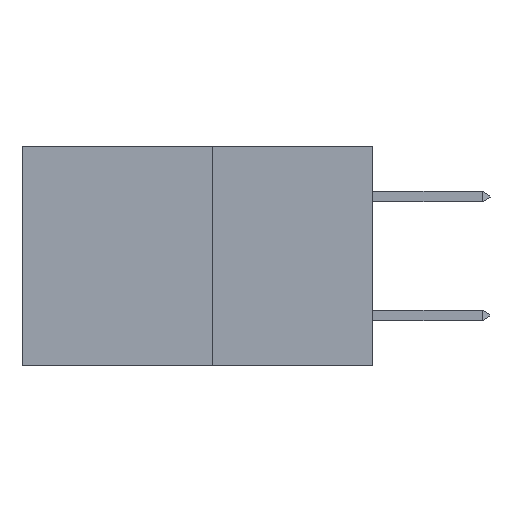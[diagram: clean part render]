
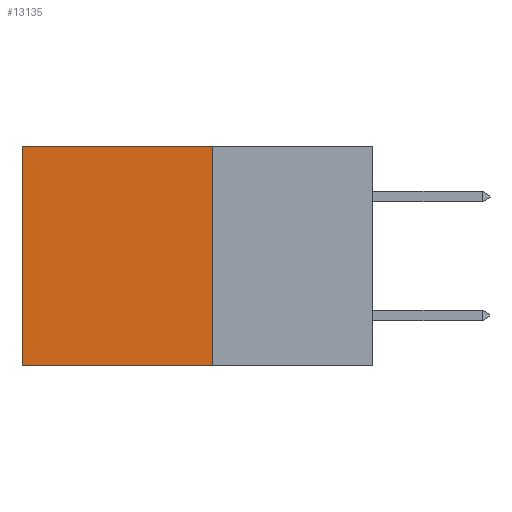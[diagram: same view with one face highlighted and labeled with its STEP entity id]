
A CAD part, left-side view. The second image highlights one B-rep face of the part: STEP entity #13135.
In plain terms, the highlighted planar face has unit normal (-1, 0, 0).
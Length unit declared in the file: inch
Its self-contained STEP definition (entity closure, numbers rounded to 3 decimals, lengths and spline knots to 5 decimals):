
#184 = ORIENTED_EDGE ( 'NONE', *, *, #9092, .T. ) ;
#260 = EDGE_LOOP ( 'NONE', ( #825, #1662, #6751, #184 ) ) ;
#454 = CARTESIAN_POINT ( 'NONE',  ( 0.277, 0.27, -0.37 ) ) ;
#545 = CARTESIAN_POINT ( 'NONE',  ( 0.277, 0.27, 0. ) ) ;
#825 = ORIENTED_EDGE ( 'NONE', *, *, #13621, .T. ) ;
#1633 = VECTOR ( 'NONE', #1637, 39.37008 ) ;
#1634 = VERTEX_POINT ( 'NONE', #9006 ) ;
#1637 = DIRECTION ( 'NONE',  ( 0., 0., -1. ) ) ;
#1662 = ORIENTED_EDGE ( 'NONE', *, *, #13455, .F. ) ;
#3047 = VERTEX_POINT ( 'NONE', #545 ) ;
#3862 = EDGE_CURVE ( 'NONE', #3047, #8270, #4620, .T. ) ;
#4149 = CARTESIAN_POINT ( 'NONE',  ( 0.277, 0.59, -0.37 ) ) ;
#4620 = LINE ( 'NONE', #454, #11533 ) ;
#5088 = LINE ( 'NONE', #4149, #1633 ) ;
#6734 = FACE_OUTER_BOUND ( 'NONE', #260, .T. ) ;
#6751 = ORIENTED_EDGE ( 'NONE', *, *, #3862, .F. ) ;
#7957 = DIRECTION ( 'NONE',  ( 0., 1., 0. ) ) ;
#8270 = VERTEX_POINT ( 'NONE', #9185 ) ;
#8368 = DIRECTION ( 'NONE',  ( 0., 0., -1. ) ) ;
#8932 = AXIS2_PLACEMENT_3D ( 'NONE', #14796, #16027, #8368 ) ;
#9006 = CARTESIAN_POINT ( 'NONE',  ( 0.277, 0.59, 0. ) ) ;
#9092 = EDGE_CURVE ( 'NONE', #3047, #1634, #11750, .T. ) ;
#9103 = CARTESIAN_POINT ( 'NONE',  ( 0.277, 0.27, -0.37 ) ) ;
#9185 = CARTESIAN_POINT ( 'NONE',  ( 0.277, 0.27, -0.37 ) ) ;
#11198 = DIRECTION ( 'NONE',  ( 0., 0., -1. ) ) ;
#11341 = VECTOR ( 'NONE', #7957, 39.37008 ) ;
#11408 = VECTOR ( 'NONE', #13010, 39.37008 ) ;
#11533 = VECTOR ( 'NONE', #11198, 39.37008 ) ;
#11750 = LINE ( 'NONE', #15652, #11341 ) ;
#11817 = LINE ( 'NONE', #9103, #11408 ) ;
#11872 = CARTESIAN_POINT ( 'NONE',  ( 0.277, 0.59, -0.37 ) ) ;
#12228 = PLANE ( 'NONE',  #8932 ) ;
#13010 = DIRECTION ( 'NONE',  ( 0., 1., 0. ) ) ;
#13135 = ADVANCED_FACE ( 'NONE', ( #6734 ), #12228, .F. ) ;
#13455 = EDGE_CURVE ( 'NONE', #8270, #13540, #11817, .T. ) ;
#13540 = VERTEX_POINT ( 'NONE', #11872 ) ;
#13621 = EDGE_CURVE ( 'NONE', #1634, #13540, #5088, .T. ) ;
#14796 = CARTESIAN_POINT ( 'NONE',  ( 0.277, 0.27, -0.37 ) ) ;
#15652 = CARTESIAN_POINT ( 'NONE',  ( 0.277, 0.27, 0. ) ) ;
#16027 = DIRECTION ( 'NONE',  ( 1., 0., 0. ) ) ;
